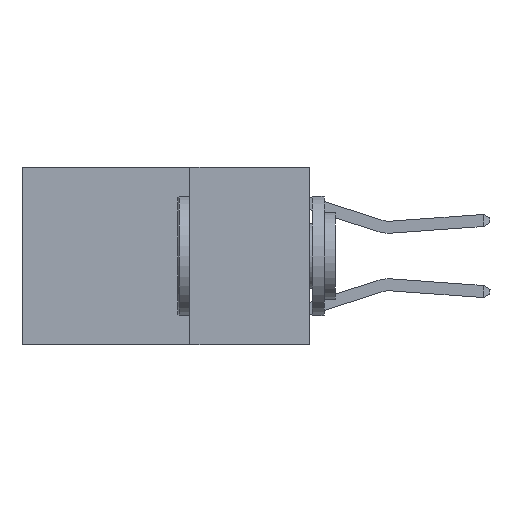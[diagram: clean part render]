
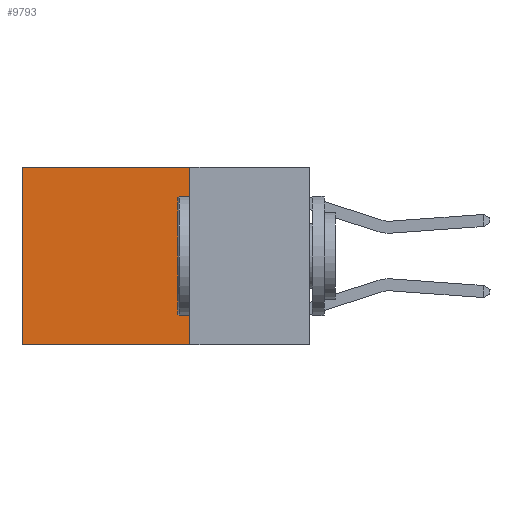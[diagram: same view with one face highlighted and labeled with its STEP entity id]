
A CAD part, left-side view. The second image highlights one B-rep face of the part: STEP entity #9793.
In plain terms, the highlighted planar face has unit normal (-1, 0, 0).
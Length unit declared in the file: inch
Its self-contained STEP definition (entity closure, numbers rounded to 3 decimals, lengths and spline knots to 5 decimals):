
#296 = EDGE_CURVE ( 'NONE', #2032, #12884, #9137, .T. ) ;
#605 = EDGE_CURVE ( 'NONE', #6246, #15589, #1907, .T. ) ;
#782 = ORIENTED_EDGE ( 'NONE', *, *, #296, .F. ) ;
#926 = ORIENTED_EDGE ( 'NONE', *, *, #14404, .F. ) ;
#1211 = CARTESIAN_POINT ( 'NONE',  ( 0.2625, 0.6, 0. ) ) ;
#1219 = DIRECTION ( 'NONE',  ( 0., 1., 0. ) ) ;
#1334 = ORIENTED_EDGE ( 'NONE', *, *, #605, .T. ) ;
#1865 = FACE_OUTER_BOUND ( 'NONE', #3951, .T. ) ;
#1907 = LINE ( 'NONE', #14834, #15389 ) ;
#2032 = VERTEX_POINT ( 'NONE', #11114 ) ;
#2033 = EDGE_CURVE ( 'NONE', #2032, #6246, #12723, .T. ) ;
#2901 = DIRECTION ( 'NONE',  ( 0., 0., -1. ) ) ;
#2990 = PLANE ( 'NONE',  #8508 ) ;
#3920 = LINE ( 'NONE', #6114, #9218 ) ;
#3951 = EDGE_LOOP ( 'NONE', ( #1334, #926, #782, #10905 ) ) ;
#4263 = DIRECTION ( 'NONE',  ( 0., 0., -1. ) ) ;
#5348 = CARTESIAN_POINT ( 'NONE',  ( 0.2625, 0.25, 0. ) ) ;
#6114 = CARTESIAN_POINT ( 'NONE',  ( 0.2625, 0.25, -0.37 ) ) ;
#6221 = CARTESIAN_POINT ( 'NONE',  ( 0.2625, 0.25, 0. ) ) ;
#6246 = VERTEX_POINT ( 'NONE', #1211 ) ;
#6409 = CARTESIAN_POINT ( 'NONE',  ( 0.2625, 0.6, -0.37 ) ) ;
#8508 = AXIS2_PLACEMENT_3D ( 'NONE', #9237, #10524, #4263 ) ;
#9137 = LINE ( 'NONE', #5348, #9321 ) ;
#9218 = VECTOR ( 'NONE', #1219, 39.37008 ) ;
#9237 = CARTESIAN_POINT ( 'NONE',  ( 0.2625, 0.25, 0. ) ) ;
#9321 = VECTOR ( 'NONE', #2901, 39.37008 ) ;
#9727 = DIRECTION ( 'NONE',  ( 0., 1., 0. ) ) ;
#9793 = ADVANCED_FACE ( 'NONE', ( #1865 ), #2990, .F. ) ;
#10524 = DIRECTION ( 'NONE',  ( 1., 0., 0. ) ) ;
#10905 = ORIENTED_EDGE ( 'NONE', *, *, #2033, .T. ) ;
#11114 = CARTESIAN_POINT ( 'NONE',  ( 0.2625, 0.25, 0. ) ) ;
#12427 = CARTESIAN_POINT ( 'NONE',  ( 0.2625, 0.25, -0.37 ) ) ;
#12723 = LINE ( 'NONE', #6221, #14393 ) ;
#12884 = VERTEX_POINT ( 'NONE', #12427 ) ;
#14393 = VECTOR ( 'NONE', #9727, 39.37008 ) ;
#14404 = EDGE_CURVE ( 'NONE', #12884, #15589, #3920, .T. ) ;
#14834 = CARTESIAN_POINT ( 'NONE',  ( 0.2625, 0.6, 0. ) ) ;
#15051 = DIRECTION ( 'NONE',  ( 0., 0., -1. ) ) ;
#15389 = VECTOR ( 'NONE', #15051, 39.37008 ) ;
#15589 = VERTEX_POINT ( 'NONE', #6409 ) ;
